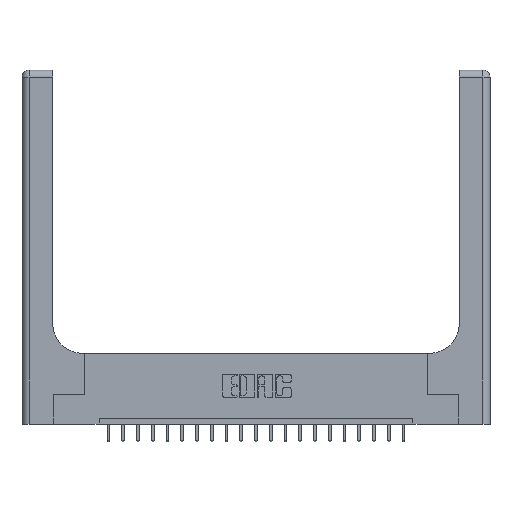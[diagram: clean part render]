
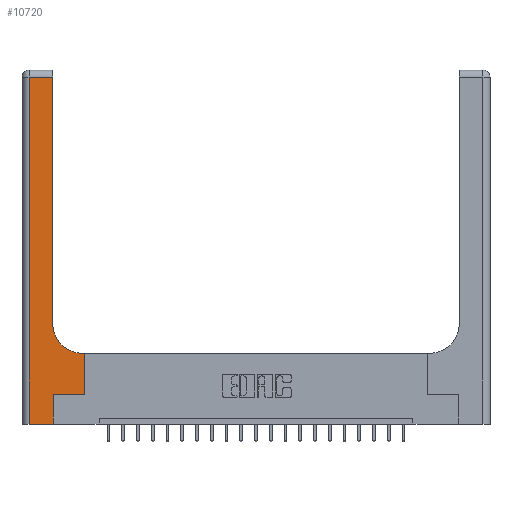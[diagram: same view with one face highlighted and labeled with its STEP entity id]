
A CAD part, top view. The second image highlights one B-rep face of the part: STEP entity #10720.
In plain terms, the highlighted planar face has unit normal (0, 0, 1).
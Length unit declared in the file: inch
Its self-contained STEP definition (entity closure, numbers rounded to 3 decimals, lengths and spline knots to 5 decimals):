
#347 = ORIENTED_EDGE ( 'NONE', *, *, #6215, .T. ) ;
#489 = CIRCLE ( 'NONE', #13613, 0.25 ) ;
#523 = ORIENTED_EDGE ( 'NONE', *, *, #8999, .T. ) ;
#606 = ORIENTED_EDGE ( 'NONE', *, *, #3482, .T. ) ;
#803 = CARTESIAN_POINT ( 'NONE',  ( 0.26, 0.6, 0.37 ) ) ;
#1245 = VECTOR ( 'NONE', #13247, 39.37008 ) ;
#1408 = AXIS2_PLACEMENT_3D ( 'NONE', #3673, #11905, #10475 ) ;
#1434 = DIRECTION ( 'NONE',  ( 0., 1., 0. ) ) ;
#1553 = LINE ( 'NONE', #6270, #12782 ) ;
#1584 = CARTESIAN_POINT ( 'NONE',  ( 0.528, 0.25, 0.37 ) ) ;
#2958 = ORIENTED_EDGE ( 'NONE', *, *, #6010, .T. ) ;
#3156 = VERTEX_POINT ( 'NONE', #12295 ) ;
#3224 = CARTESIAN_POINT ( 'NONE',  ( 0.26, 3., 0.37 ) ) ;
#3231 = LINE ( 'NONE', #13381, #21026 ) ;
#3482 = EDGE_CURVE ( 'NONE', #4226, #8537, #19130, .T. ) ;
#3673 = CARTESIAN_POINT ( 'NONE',  ( 0., 3., 0.37 ) ) ;
#3846 = CARTESIAN_POINT ( 'NONE',  ( 0.06, 2.94, 0.37 ) ) ;
#4226 = VERTEX_POINT ( 'NONE', #7343 ) ;
#4541 = VERTEX_POINT ( 'NONE', #9698 ) ;
#4624 = VECTOR ( 'NONE', #1434, 39.37008 ) ;
#4634 = DIRECTION ( 'NONE',  ( 1., 0., 0. ) ) ;
#4696 = ORIENTED_EDGE ( 'NONE', *, *, #11844, .T. ) ;
#5515 = ORIENTED_EDGE ( 'NONE', *, *, #7229, .T. ) ;
#5674 = ORIENTED_EDGE ( 'NONE', *, *, #16099, .T. ) ;
#5685 = VECTOR ( 'NONE', #13843, 39.37008 ) ;
#6010 = EDGE_CURVE ( 'NONE', #3156, #4226, #489, .T. ) ;
#6215 = EDGE_CURVE ( 'NONE', #11328, #18344, #7373, .T. ) ;
#6270 = CARTESIAN_POINT ( 'NONE',  ( 0.265, 0., 0.37 ) ) ;
#6618 = VERTEX_POINT ( 'NONE', #3846 ) ;
#6723 = CARTESIAN_POINT ( 'NONE',  ( 0.528, 0.25, 0.37 ) ) ;
#7229 = EDGE_CURVE ( 'NONE', #8537, #6618, #3231, .T. ) ;
#7236 = DIRECTION ( 'NONE',  ( 0., 0., -1. ) ) ;
#7343 = CARTESIAN_POINT ( 'NONE',  ( 0.26, 0.85, 0.37 ) ) ;
#7373 = LINE ( 'NONE', #7651, #14485 ) ;
#7644 = VERTEX_POINT ( 'NONE', #1584 ) ;
#7651 = CARTESIAN_POINT ( 'NONE',  ( 0., 0., 0.37 ) ) ;
#7755 = LINE ( 'NONE', #20017, #20213 ) ;
#8537 = VERTEX_POINT ( 'NONE', #17066 ) ;
#8930 = EDGE_CURVE ( 'NONE', #16907, #7644, #7755, .T. ) ;
#8999 = EDGE_CURVE ( 'NONE', #4541, #3156, #13858, .T. ) ;
#9698 = CARTESIAN_POINT ( 'NONE',  ( 0.528, 0.6, 0.37 ) ) ;
#10258 = DIRECTION ( 'NONE',  ( 1., 0., 0. ) ) ;
#10475 = DIRECTION ( 'NONE',  ( -1., 0., 0. ) ) ;
#10718 = VECTOR ( 'NONE', #11702, 39.37008 ) ;
#10720 = ADVANCED_FACE ( 'NONE', ( #20637 ), #18498, .F. ) ;
#11328 = VERTEX_POINT ( 'NONE', #14964 ) ;
#11702 = DIRECTION ( 'NONE',  ( 0., 1., 0. ) ) ;
#11844 = EDGE_CURVE ( 'NONE', #6618, #11328, #15026, .T. ) ;
#11905 = DIRECTION ( 'NONE',  ( 0., 0., -1. ) ) ;
#12295 = CARTESIAN_POINT ( 'NONE',  ( 0.51, 0.6, 0.37 ) ) ;
#12570 = DIRECTION ( 'NONE',  ( 0., 1., 0. ) ) ;
#12782 = VECTOR ( 'NONE', #12570, 39.37008 ) ;
#13247 = DIRECTION ( 'NONE',  ( 0., -1., 0. ) ) ;
#13381 = CARTESIAN_POINT ( 'NONE',  ( 0., 2.94, 0.37 ) ) ;
#13427 = CARTESIAN_POINT ( 'NONE',  ( 0.51, 0.85, 0.37 ) ) ;
#13613 = AXIS2_PLACEMENT_3D ( 'NONE', #13427, #7236, #16814 ) ;
#13810 = EDGE_LOOP ( 'NONE', ( #606, #5515, #4696, #347, #5674, #16722, #14928, #523, #2958 ) ) ;
#13843 = DIRECTION ( 'NONE',  ( -1., 0., 0. ) ) ;
#13858 = LINE ( 'NONE', #803, #5685 ) ;
#14485 = VECTOR ( 'NONE', #4634, 39.37008 ) ;
#14928 = ORIENTED_EDGE ( 'NONE', *, *, #17863, .T. ) ;
#14964 = CARTESIAN_POINT ( 'NONE',  ( 0.06, 0., 0.37 ) ) ;
#15026 = LINE ( 'NONE', #19616, #1245 ) ;
#16099 = EDGE_CURVE ( 'NONE', #18344, #16907, #1553, .T. ) ;
#16722 = ORIENTED_EDGE ( 'NONE', *, *, #8930, .T. ) ;
#16814 = DIRECTION ( 'NONE',  ( 1., 0., 0. ) ) ;
#16907 = VERTEX_POINT ( 'NONE', #16992 ) ;
#16992 = CARTESIAN_POINT ( 'NONE',  ( 0.265, 0.25, 0.37 ) ) ;
#17066 = CARTESIAN_POINT ( 'NONE',  ( 0.26, 2.94, 0.37 ) ) ;
#17353 = CARTESIAN_POINT ( 'NONE',  ( 0.265, 0., 0.37 ) ) ;
#17863 = EDGE_CURVE ( 'NONE', #7644, #4541, #20153, .T. ) ;
#18312 = DIRECTION ( 'NONE',  ( -1., 0., 0. ) ) ;
#18344 = VERTEX_POINT ( 'NONE', #17353 ) ;
#18498 = PLANE ( 'NONE',  #1408 ) ;
#19130 = LINE ( 'NONE', #3224, #4624 ) ;
#19616 = CARTESIAN_POINT ( 'NONE',  ( 0.06, 3., 0.37 ) ) ;
#20017 = CARTESIAN_POINT ( 'NONE',  ( 0.265, 0.25, 0.37 ) ) ;
#20153 = LINE ( 'NONE', #6723, #10718 ) ;
#20213 = VECTOR ( 'NONE', #10258, 39.37008 ) ;
#20637 = FACE_OUTER_BOUND ( 'NONE', #13810, .T. ) ;
#21026 = VECTOR ( 'NONE', #18312, 39.37008 ) ;
